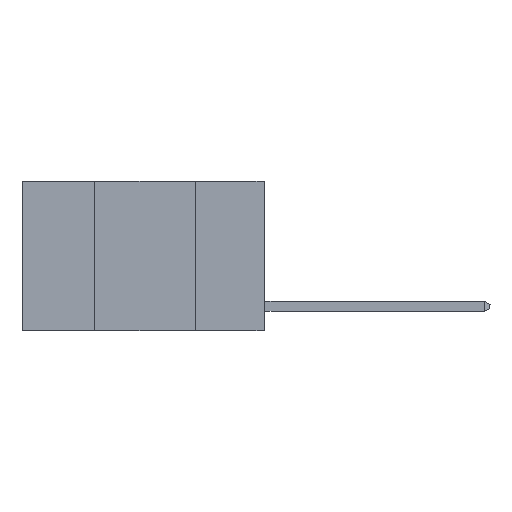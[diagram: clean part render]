
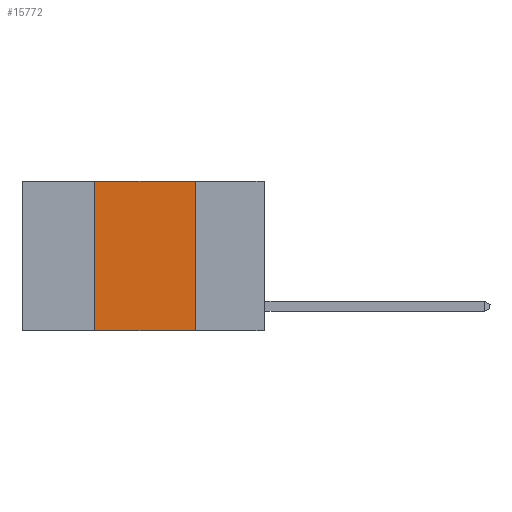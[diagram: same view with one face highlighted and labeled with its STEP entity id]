
A CAD part, left-side view. The second image highlights one B-rep face of the part: STEP entity #15772.
In plain terms, the highlighted planar face has unit normal (-1, 0, 0).
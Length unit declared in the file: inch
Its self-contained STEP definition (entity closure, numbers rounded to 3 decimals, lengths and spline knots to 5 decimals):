
#35 = AXIS2_PLACEMENT_3D ( 'NONE', #5288, #15295, #7794 ) ;
#242 = ORIENTED_EDGE ( 'NONE', *, *, #749, .F. ) ;
#704 = CARTESIAN_POINT ( 'NONE',  ( 0., 0.6, 0. ) ) ;
#749 = EDGE_CURVE ( 'NONE', #3765, #8847, #2044, .T. ) ;
#781 = DIRECTION ( 'NONE',  ( 0., 0., -1. ) ) ;
#954 = VECTOR ( 'NONE', #3247, 39.37008 ) ;
#1349 = LINE ( 'NONE', #704, #954 ) ;
#2044 = LINE ( 'NONE', #9526, #4997 ) ;
#2621 = VECTOR ( 'NONE', #9436, 39.37008 ) ;
#2970 = CARTESIAN_POINT ( 'NONE',  ( 0., 0.42, -0.37 ) ) ;
#3247 = DIRECTION ( 'NONE',  ( 0., -1., 0. ) ) ;
#3765 = VERTEX_POINT ( 'NONE', #10389 ) ;
#4303 = CARTESIAN_POINT ( 'NONE',  ( 0., 0.6, -0.37 ) ) ;
#4997 = VECTOR ( 'NONE', #781, 39.37008 ) ;
#5094 = VERTEX_POINT ( 'NONE', #2970 ) ;
#5288 = CARTESIAN_POINT ( 'NONE',  ( 0., 0.6, 0. ) ) ;
#5928 = LINE ( 'NONE', #14428, #2621 ) ;
#6261 = CARTESIAN_POINT ( 'NONE',  ( 0., 0.17, -0.37 ) ) ;
#6507 = EDGE_CURVE ( 'NONE', #7845, #3765, #1349, .T. ) ;
#6661 = ORIENTED_EDGE ( 'NONE', *, *, #6507, .F. ) ;
#7012 = LINE ( 'NONE', #4303, #14476 ) ;
#7671 = ORIENTED_EDGE ( 'NONE', *, *, #13656, .T. ) ;
#7794 = DIRECTION ( 'NONE',  ( 0., 0., -1. ) ) ;
#7845 = VERTEX_POINT ( 'NONE', #9675 ) ;
#8847 = VERTEX_POINT ( 'NONE', #6261 ) ;
#9284 = EDGE_LOOP ( 'NONE', ( #242, #6661, #11999, #7671 ) ) ;
#9436 = DIRECTION ( 'NONE',  ( 0., 0., 1. ) ) ;
#9526 = CARTESIAN_POINT ( 'NONE',  ( 0., 0.17, 0. ) ) ;
#9675 = CARTESIAN_POINT ( 'NONE',  ( 0., 0.42, 0. ) ) ;
#10015 = FACE_OUTER_BOUND ( 'NONE', #9284, .T. ) ;
#10389 = CARTESIAN_POINT ( 'NONE',  ( 0., 0.17, 0. ) ) ;
#11999 = ORIENTED_EDGE ( 'NONE', *, *, #15336, .F. ) ;
#12775 = PLANE ( 'NONE',  #35 ) ;
#13040 = DIRECTION ( 'NONE',  ( 0., -1., 0. ) ) ;
#13656 = EDGE_CURVE ( 'NONE', #5094, #8847, #7012, .T. ) ;
#14428 = CARTESIAN_POINT ( 'NONE',  ( 0., 0.42, 0. ) ) ;
#14476 = VECTOR ( 'NONE', #13040, 39.37008 ) ;
#15295 = DIRECTION ( 'NONE',  ( 1., 0., 0. ) ) ;
#15336 = EDGE_CURVE ( 'NONE', #5094, #7845, #5928, .T. ) ;
#15772 = ADVANCED_FACE ( 'NONE', ( #10015 ), #12775, .F. ) ;
